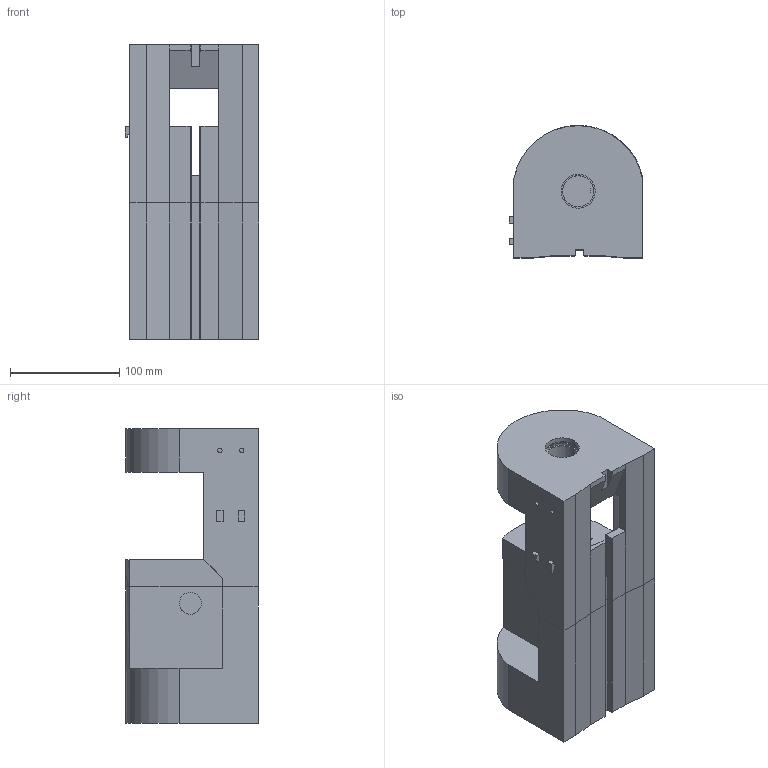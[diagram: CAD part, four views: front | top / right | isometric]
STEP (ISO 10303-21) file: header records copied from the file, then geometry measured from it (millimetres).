
FILE_DESCRIPTION (( 'STEP AP214' ), '1' );
FILE_NAME ('Reciver.STEP', '2025-05-18T10:37:44', ( '' ), ( '' ), 'SwSTEP 2.0', 'SolidWorks 2024', '' );
FILE_SCHEMA (( 'AUTOMOTIVE_DESIGN' ));
Length unit declared in the file: millimetre
Products named in the file (1): Reciver
Bounding box: 121.82 x 121 x 270 mm (x, y, z)
Volume: 2205982.3 mm3; surface area: 197489.7 mm2
Topology: 2 solids, 2 shells, 167 faces, 434 edges, 286 vertices
Faces by surface type: plane 96, cylinder 67, cone 4
Entity records: 5411 total; most frequent: CARTESIAN_POINT 1103, DIRECTION 908, ORIENTED_EDGE 868, EDGE_CURVE 434, AXIS2_PLACEMENT_3D 317, VERTEX_POINT 286, LINE 274, VECTOR 274
